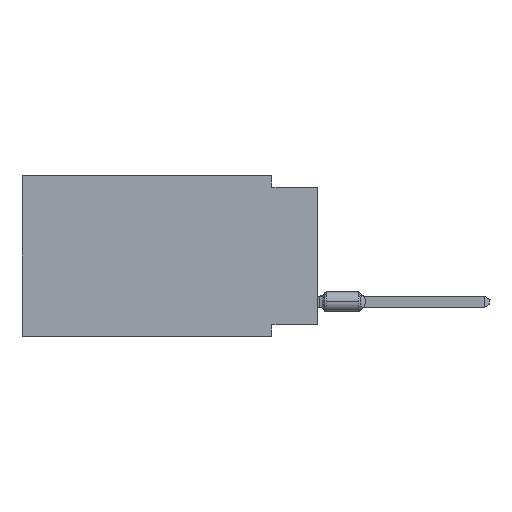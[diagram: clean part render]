
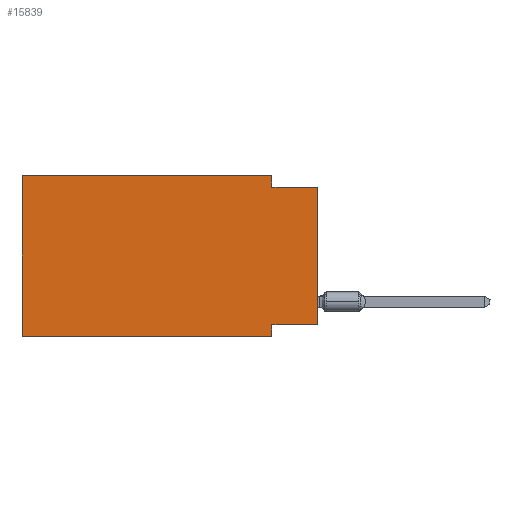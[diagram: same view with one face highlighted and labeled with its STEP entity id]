
A CAD part, left-side view. The second image highlights one B-rep face of the part: STEP entity #15839.
In plain terms, the highlighted planar face has unit normal (-1, 0, 0).
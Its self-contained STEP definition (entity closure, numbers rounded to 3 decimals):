
#68 = ORIENTED_EDGE ( 'NONE', *, *, #84787, .F. ) ;
#3529 = VECTOR ( 'NONE', #19052, 1000. ) ;
#5180 = VECTOR ( 'NONE', #110618, 1000. ) ;
#6975 = VERTEX_POINT ( 'NONE', #29386 ) ;
#8012 = DIRECTION ( 'NONE',  ( 0., -1., 0. ) ) ;
#12677 = ORIENTED_EDGE ( 'NONE', *, *, #51064, .F. ) ;
#13246 = VERTEX_POINT ( 'NONE', #32504 ) ;
#14819 = VERTEX_POINT ( 'NONE', #48113 ) ;
#15839 = ADVANCED_FACE ( 'NONE', ( #79626 ), #31986, .F. ) ;
#19052 = DIRECTION ( 'NONE',  ( 0., -1., 0. ) ) ;
#19357 = EDGE_CURVE ( 'NONE', #118724, #13246, #55273, .T. ) ;
#20337 = CARTESIAN_POINT ( 'NONE',  ( 0., 2.54, -8.89 ) ) ;
#22547 = VECTOR ( 'NONE', #53483, 1000. ) ;
#24720 = CARTESIAN_POINT ( 'NONE',  ( 0., 2.54, -8.255 ) ) ;
#25318 = VECTOR ( 'NONE', #92072, 1000. ) ;
#26188 = ORIENTED_EDGE ( 'NONE', *, *, #49031, .F. ) ;
#29154 = LINE ( 'NONE', #56904, #5180 ) ;
#29386 = CARTESIAN_POINT ( 'NONE',  ( 0., 2.54, -0.635 ) ) ;
#29689 = DIRECTION ( 'NONE',  ( 0., 0., 1. ) ) ;
#31986 = PLANE ( 'NONE',  #85484 ) ;
#32504 = CARTESIAN_POINT ( 'NONE',  ( 0., 2.54, -8.89 ) ) ;
#34359 = CARTESIAN_POINT ( 'NONE',  ( 0., 16.383, 0. ) ) ;
#35880 = ORIENTED_EDGE ( 'NONE', *, *, #86882, .F. ) ;
#36954 = ORIENTED_EDGE ( 'NONE', *, *, #19357, .T. ) ;
#38458 = LINE ( 'NONE', #20337, #88469 ) ;
#41404 = DIRECTION ( 'NONE',  ( 0., 1., 0. ) ) ;
#42318 = CARTESIAN_POINT ( 'NONE',  ( 0., 16.383, -8.89 ) ) ;
#42846 = DIRECTION ( 'NONE',  ( 0., 0., -1. ) ) ;
#47085 = VECTOR ( 'NONE', #29689, 1000. ) ;
#48113 = CARTESIAN_POINT ( 'NONE',  ( 0., 0., -0.635 ) ) ;
#49031 = EDGE_CURVE ( 'NONE', #78662, #6975, #108421, .T. ) ;
#51064 = EDGE_CURVE ( 'NONE', #6975, #14819, #55857, .T. ) ;
#53279 = CARTESIAN_POINT ( 'NONE',  ( 0., 16.383, 0. ) ) ;
#53483 = DIRECTION ( 'NONE',  ( 0., -1., 0. ) ) ;
#55273 = LINE ( 'NONE', #64890, #3529 ) ;
#55289 = CARTESIAN_POINT ( 'NONE',  ( 0., 2.54, 0. ) ) ;
#55401 = VECTOR ( 'NONE', #41404, 1000. ) ;
#55857 = LINE ( 'NONE', #99919, #22547 ) ;
#56904 = CARTESIAN_POINT ( 'NONE',  ( 0., 0., 0. ) ) ;
#58885 = LINE ( 'NONE', #96284, #55401 ) ;
#64813 = ORIENTED_EDGE ( 'NONE', *, *, #109199, .F. ) ;
#64890 = CARTESIAN_POINT ( 'NONE',  ( 0., 16.383, -8.89 ) ) ;
#65737 = CARTESIAN_POINT ( 'NONE',  ( 0., 16.383, 0. ) ) ;
#67950 = CARTESIAN_POINT ( 'NONE',  ( 0., 2.54, 0. ) ) ;
#68326 = VECTOR ( 'NONE', #8012, 1000. ) ;
#71380 = LINE ( 'NONE', #53279, #68326 ) ;
#72319 = ORIENTED_EDGE ( 'NONE', *, *, #79495, .F. ) ;
#74422 = EDGE_LOOP ( 'NONE', ( #79440, #12677, #26188, #64813, #72319, #36954, #35880, #68 ) ) ;
#75855 = DIRECTION ( 'NONE',  ( 0., 0., -1. ) ) ;
#78414 = DIRECTION ( 'NONE',  ( 1., 0., 0. ) ) ;
#78662 = VERTEX_POINT ( 'NONE', #67950 ) ;
#79440 = ORIENTED_EDGE ( 'NONE', *, *, #92594, .T. ) ;
#79495 = EDGE_CURVE ( 'NONE', #118724, #109667, #84573, .T. ) ;
#79626 = FACE_OUTER_BOUND ( 'NONE', #74422, .T. ) ;
#82799 = VERTEX_POINT ( 'NONE', #24720 ) ;
#84573 = LINE ( 'NONE', #111742, #47085 ) ;
#84787 = EDGE_CURVE ( 'NONE', #119284, #82799, #58885, .T. ) ;
#85484 = AXIS2_PLACEMENT_3D ( 'NONE', #34359, #78414, #42846 ) ;
#86882 = EDGE_CURVE ( 'NONE', #82799, #13246, #38458, .T. ) ;
#88469 = VECTOR ( 'NONE', #75855, 1000. ) ;
#92072 = DIRECTION ( 'NONE',  ( 0., 0., -1. ) ) ;
#92594 = EDGE_CURVE ( 'NONE', #119284, #14819, #29154, .T. ) ;
#96284 = CARTESIAN_POINT ( 'NONE',  ( 0., 0., -8.255 ) ) ;
#99919 = CARTESIAN_POINT ( 'NONE',  ( 0., 0., -0.635 ) ) ;
#108421 = LINE ( 'NONE', #55289, #25318 ) ;
#108485 = CARTESIAN_POINT ( 'NONE',  ( 0., 0., -8.255 ) ) ;
#109199 = EDGE_CURVE ( 'NONE', #109667, #78662, #71380, .T. ) ;
#109667 = VERTEX_POINT ( 'NONE', #65737 ) ;
#110618 = DIRECTION ( 'NONE',  ( 0., 0., 1. ) ) ;
#111742 = CARTESIAN_POINT ( 'NONE',  ( 0., 16.383, 0. ) ) ;
#118724 = VERTEX_POINT ( 'NONE', #42318 ) ;
#119284 = VERTEX_POINT ( 'NONE', #108485 ) ;
